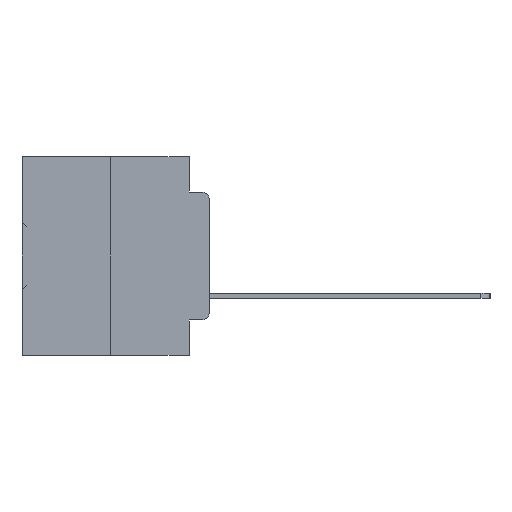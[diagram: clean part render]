
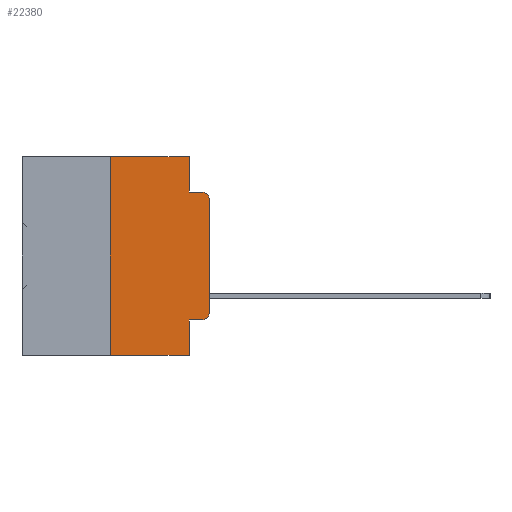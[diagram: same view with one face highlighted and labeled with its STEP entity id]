
A CAD part, left-side view. The second image highlights one B-rep face of the part: STEP entity #22380.
In plain terms, the highlighted planar face has unit normal (-1, 0, 0).
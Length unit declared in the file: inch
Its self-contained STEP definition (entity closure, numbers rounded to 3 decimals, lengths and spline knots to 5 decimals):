
#918 = LINE ( 'NONE', #1926, #22472 ) ;
#1168 = VECTOR ( 'NONE', #20057, 39.37008 ) ;
#1312 = DIRECTION ( 'NONE',  ( 0., 0., 1. ) ) ;
#1506 = CARTESIAN_POINT ( 'NONE',  ( 0., 0.473, -0.5 ) ) ;
#1926 = CARTESIAN_POINT ( 'NONE',  ( 0., 0.051, 0. ) ) ;
#2269 = CARTESIAN_POINT ( 'NONE',  ( 0., 0.25, 0. ) ) ;
#2541 = VERTEX_POINT ( 'NONE', #34060 ) ;
#3560 = CARTESIAN_POINT ( 'NONE',  ( 0., 0., -0.1085 ) ) ;
#3572 = CARTESIAN_POINT ( 'NONE',  ( 0., 0., -0.3915 ) ) ;
#3663 = EDGE_CURVE ( 'NONE', #25820, #17395, #918, .T. ) ;
#3910 = AXIS2_PLACEMENT_3D ( 'NONE', #10076, #30425, #13020 ) ;
#4314 = CARTESIAN_POINT ( 'NONE',  ( 0., 0.25, 0. ) ) ;
#4522 = DIRECTION ( 'NONE',  ( 0., -1., 0. ) ) ;
#5429 = EDGE_CURVE ( 'NONE', #31424, #33288, #28727, .T. ) ;
#7179 = AXIS2_PLACEMENT_3D ( 'NONE', #8004, #28342, #10934 ) ;
#8004 = CARTESIAN_POINT ( 'NONE',  ( 0., 0.473, 0. ) ) ;
#9048 = LINE ( 'NONE', #11275, #1168 ) ;
#9812 = VECTOR ( 'NONE', #13731, 39.37008 ) ;
#10076 = CARTESIAN_POINT ( 'NONE',  ( 0., 0.02, -0.3915 ) ) ;
#10153 = LINE ( 'NONE', #32279, #16090 ) ;
#10295 = DIRECTION ( 'NONE',  ( -1., 0., 0. ) ) ;
#10394 = CARTESIAN_POINT ( 'NONE',  ( 0., 0.25, -0.5 ) ) ;
#10934 = DIRECTION ( 'NONE',  ( 0., 0., -1. ) ) ;
#11275 = CARTESIAN_POINT ( 'NONE',  ( 0., 0.051, -0.0885 ) ) ;
#11897 = VERTEX_POINT ( 'NONE', #16372 ) ;
#12197 = VERTEX_POINT ( 'NONE', #23533 ) ;
#13020 = DIRECTION ( 'NONE',  ( 0., 0., -1. ) ) ;
#13154 = ORIENTED_EDGE ( 'NONE', *, *, #5429, .T. ) ;
#13673 = ORIENTED_EDGE ( 'NONE', *, *, #17946, .T. ) ;
#13731 = DIRECTION ( 'NONE',  ( 0., 0., -1. ) ) ;
#14196 = FACE_OUTER_BOUND ( 'NONE', #18586, .T. ) ;
#14696 = VECTOR ( 'NONE', #1312, 39.37008 ) ;
#15119 = VECTOR ( 'NONE', #34609, 39.37008 ) ;
#15500 = EDGE_CURVE ( 'NONE', #25094, #34589, #30165, .T. ) ;
#16090 = VECTOR ( 'NONE', #26389, 39.37008 ) ;
#16372 = CARTESIAN_POINT ( 'NONE',  ( 0., 0.02, -0.0885 ) ) ;
#16743 = ORIENTED_EDGE ( 'NONE', *, *, #25199, .F. ) ;
#16782 = ORIENTED_EDGE ( 'NONE', *, *, #31088, .F. ) ;
#16950 = LINE ( 'NONE', #31704, #15119 ) ;
#17395 = VERTEX_POINT ( 'NONE', #19266 ) ;
#17946 = EDGE_CURVE ( 'NONE', #33288, #11897, #34933, .T. ) ;
#18531 = ORIENTED_EDGE ( 'NONE', *, *, #29786, .T. ) ;
#18586 = EDGE_LOOP ( 'NONE', ( #13154, #13673, #16782, #16743, #21117, #20568, #20495, #19801, #19220, #18531 ) ) ;
#19220 = ORIENTED_EDGE ( 'NONE', *, *, #29836, .T. ) ;
#19266 = CARTESIAN_POINT ( 'NONE',  ( 0., 0.051, -0.5 ) ) ;
#19801 = ORIENTED_EDGE ( 'NONE', *, *, #3663, .F. ) ;
#20015 = AXIS2_PLACEMENT_3D ( 'NONE', #27682, #10295, #30649 ) ;
#20057 = DIRECTION ( 'NONE',  ( 0., -1., 0. ) ) ;
#20466 = EDGE_CURVE ( 'NONE', #25094, #17395, #36551, .T. ) ;
#20495 = ORIENTED_EDGE ( 'NONE', *, *, #20466, .T. ) ;
#20568 = ORIENTED_EDGE ( 'NONE', *, *, #15500, .F. ) ;
#20784 = EDGE_CURVE ( 'NONE', #34589, #12197, #10153, .T. ) ;
#21013 = VECTOR ( 'NONE', #30799, 39.37008 ) ;
#21117 = ORIENTED_EDGE ( 'NONE', *, *, #20784, .F. ) ;
#22380 = ADVANCED_FACE ( 'NONE', ( #14196 ), #34069, .F. ) ;
#22419 = DIRECTION ( 'NONE',  ( 0., 0., -1. ) ) ;
#22472 = VECTOR ( 'NONE', #22419, 39.37008 ) ;
#22854 = CARTESIAN_POINT ( 'NONE',  ( 0., 0.051, -0.4115 ) ) ;
#23533 = CARTESIAN_POINT ( 'NONE',  ( 0., 0.051, 0. ) ) ;
#23968 = CARTESIAN_POINT ( 'NONE',  ( 0., 0.02, -0.4115 ) ) ;
#25094 = VERTEX_POINT ( 'NONE', #10394 ) ;
#25199 = EDGE_CURVE ( 'NONE', #12197, #2541, #26155, .T. ) ;
#25820 = VERTEX_POINT ( 'NONE', #22854 ) ;
#26155 = LINE ( 'NONE', #36932, #9812 ) ;
#26389 = DIRECTION ( 'NONE',  ( 0., -1., 0. ) ) ;
#27682 = CARTESIAN_POINT ( 'NONE',  ( 0., 0.02, -0.1085 ) ) ;
#28342 = DIRECTION ( 'NONE',  ( 1., 0., 0. ) ) ;
#28727 = LINE ( 'NONE', #36490, #21013 ) ;
#28831 = VECTOR ( 'NONE', #4522, 39.37008 ) ;
#29018 = VERTEX_POINT ( 'NONE', #23968 ) ;
#29786 = EDGE_CURVE ( 'NONE', #29018, #31424, #32384, .T. ) ;
#29836 = EDGE_CURVE ( 'NONE', #25820, #29018, #16950, .T. ) ;
#30165 = LINE ( 'NONE', #4314, #14696 ) ;
#30425 = DIRECTION ( 'NONE',  ( -1., 0., 0. ) ) ;
#30649 = DIRECTION ( 'NONE',  ( 0., 0., -1. ) ) ;
#30799 = DIRECTION ( 'NONE',  ( 0., 0., 1. ) ) ;
#31088 = EDGE_CURVE ( 'NONE', #2541, #11897, #9048, .T. ) ;
#31424 = VERTEX_POINT ( 'NONE', #3572 ) ;
#31704 = CARTESIAN_POINT ( 'NONE',  ( 0., 0.051, -0.4115 ) ) ;
#32279 = CARTESIAN_POINT ( 'NONE',  ( 0., 0.473, 0. ) ) ;
#32384 = CIRCLE ( 'NONE', #3910, 0.02 ) ;
#33288 = VERTEX_POINT ( 'NONE', #3560 ) ;
#34060 = CARTESIAN_POINT ( 'NONE',  ( 0., 0.051, -0.0885 ) ) ;
#34069 = PLANE ( 'NONE',  #7179 ) ;
#34589 = VERTEX_POINT ( 'NONE', #2269 ) ;
#34609 = DIRECTION ( 'NONE',  ( 0., -1., 0. ) ) ;
#34933 = CIRCLE ( 'NONE', #20015, 0.02 ) ;
#36490 = CARTESIAN_POINT ( 'NONE',  ( 0., 0., 0. ) ) ;
#36551 = LINE ( 'NONE', #1506, #28831 ) ;
#36932 = CARTESIAN_POINT ( 'NONE',  ( 0., 0.051, 0. ) ) ;
